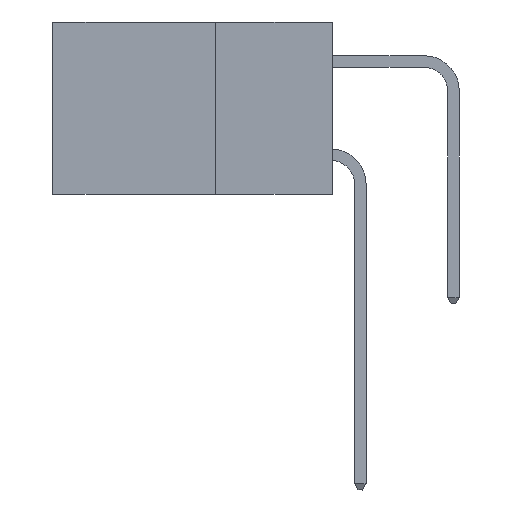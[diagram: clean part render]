
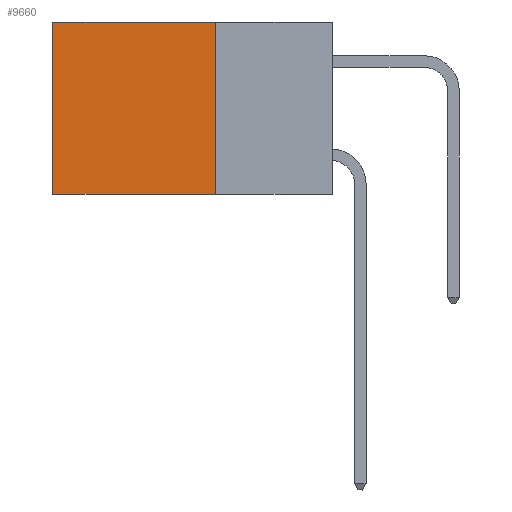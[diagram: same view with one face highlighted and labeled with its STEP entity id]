
A CAD part, left-side view. The second image highlights one B-rep face of the part: STEP entity #9660.
In plain terms, the highlighted planar face has unit normal (-1, 0, 0).
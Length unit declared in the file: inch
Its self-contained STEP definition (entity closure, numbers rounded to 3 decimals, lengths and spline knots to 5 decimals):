
#1437 = PLANE ( 'NONE',  #13398 ) ;
#2248 = CARTESIAN_POINT ( 'NONE',  ( 0.2615, 0.25, -0.37 ) ) ;
#3712 = DIRECTION ( 'NONE',  ( 0., 1., 0. ) ) ;
#4430 = CARTESIAN_POINT ( 'NONE',  ( 0.2615, 0.25, 0. ) ) ;
#6578 = VECTOR ( 'NONE', #23652, 39.37008 ) ;
#7155 = DIRECTION ( 'NONE',  ( 0., 0., -1. ) ) ;
#7389 = ORIENTED_EDGE ( 'NONE', *, *, #20729, .F. ) ;
#7411 = ORIENTED_EDGE ( 'NONE', *, *, #21349, .T. ) ;
#7451 = EDGE_LOOP ( 'NONE', ( #7411, #16164, #7389, #8330 ) ) ;
#8330 = ORIENTED_EDGE ( 'NONE', *, *, #23482, .T. ) ;
#8487 = VERTEX_POINT ( 'NONE', #8588 ) ;
#8588 = CARTESIAN_POINT ( 'NONE',  ( 0.2615, 0.6, 0. ) ) ;
#8747 = VECTOR ( 'NONE', #21193, 39.37008 ) ;
#9660 = ADVANCED_FACE ( 'NONE', ( #21494 ), #1437, .F. ) ;
#10798 = LINE ( 'NONE', #18508, #21478 ) ;
#13398 = AXIS2_PLACEMENT_3D ( 'NONE', #23551, #15967, #14505 ) ;
#13634 = VERTEX_POINT ( 'NONE', #19133 ) ;
#14505 = DIRECTION ( 'NONE',  ( 0., 0., -1. ) ) ;
#14597 = CARTESIAN_POINT ( 'NONE',  ( 0.2615, 0.25, 0. ) ) ;
#14719 = LINE ( 'NONE', #17977, #6578 ) ;
#15947 = VERTEX_POINT ( 'NONE', #4430 ) ;
#15967 = DIRECTION ( 'NONE',  ( 1., 0., 0. ) ) ;
#16164 = ORIENTED_EDGE ( 'NONE', *, *, #23573, .F. ) ;
#16230 = VECTOR ( 'NONE', #3712, 39.37008 ) ;
#17703 = LINE ( 'NONE', #21434, #8747 ) ;
#17977 = CARTESIAN_POINT ( 'NONE',  ( 0.2615, 0.25, -0.37 ) ) ;
#18342 = LINE ( 'NONE', #14597, #16230 ) ;
#18508 = CARTESIAN_POINT ( 'NONE',  ( 0.2615, 0.6, -0.37 ) ) ;
#19133 = CARTESIAN_POINT ( 'NONE',  ( 0.2615, 0.6, -0.37 ) ) ;
#20585 = VERTEX_POINT ( 'NONE', #2248 ) ;
#20729 = EDGE_CURVE ( 'NONE', #15947, #20585, #17703, .T. ) ;
#21193 = DIRECTION ( 'NONE',  ( 0., 0., -1. ) ) ;
#21349 = EDGE_CURVE ( 'NONE', #8487, #13634, #10798, .T. ) ;
#21434 = CARTESIAN_POINT ( 'NONE',  ( 0.2615, 0.25, -0.37 ) ) ;
#21478 = VECTOR ( 'NONE', #7155, 39.37008 ) ;
#21494 = FACE_OUTER_BOUND ( 'NONE', #7451, .T. ) ;
#23482 = EDGE_CURVE ( 'NONE', #15947, #8487, #18342, .T. ) ;
#23551 = CARTESIAN_POINT ( 'NONE',  ( 0.2615, 0.25, -0.37 ) ) ;
#23573 = EDGE_CURVE ( 'NONE', #20585, #13634, #14719, .T. ) ;
#23652 = DIRECTION ( 'NONE',  ( 0., 1., 0. ) ) ;
